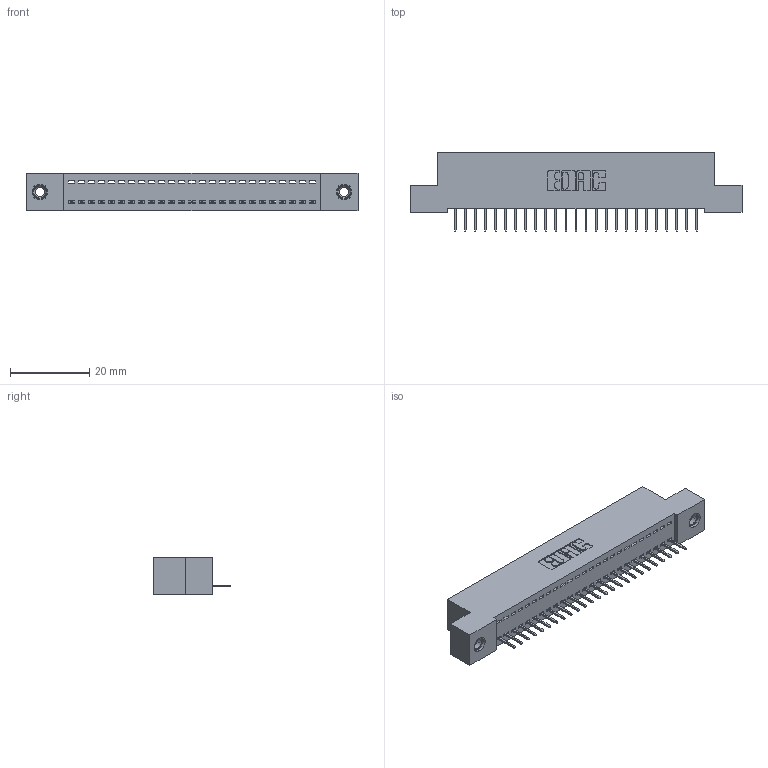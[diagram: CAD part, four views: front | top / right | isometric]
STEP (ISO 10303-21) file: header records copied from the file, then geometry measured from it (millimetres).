
FILE_DESCRIPTION (( 'STEP AP203' ), '1' );
FILE_NAME ('342-025-524-108.STEP', '2018-08-11T03:27:08', ( '' ), ( '' ), 'SwSTEP 2.0', 'SolidWorks 2016', '' );
FILE_SCHEMA (( 'CONFIG_CONTROL_DESIGN' ));
Length unit declared in the file: inch
Products named in the file (4): 342 Part_TI; 345-292-001_345-293-124; 345-250-001_345-250-003-102; 342-025-524-108
Assembly tree (28 placements, depth 2):
  342-025-524-108
    342 Part_TI
    345-292-001_345-293-124  x25
    345-250-001_345-250-003-102  x2
Bounding box: 83.82 x 19.69 x 9.4 mm (x, y, z)
Volume: 7182.3 mm3; surface area: 9940.5 mm2
Topology: 28 solids, 28 shells, 1720 faces, 4935 edges, 3182 vertices
Faces by surface type: plane 1298, cylinder 406, cone 12, torus 4
Entity records: 18610 total; most frequent: CARTESIAN_POINT 3192, ORIENTED_EDGE 3146, DIRECTION 2761, EDGE_CURVE 1573, VECTOR 1429, LINE 1429, VERTEX_POINT 1040, AXIS2_PLACEMENT_3D 666
